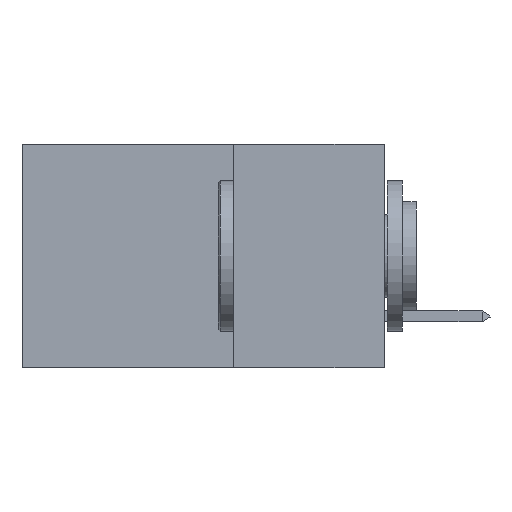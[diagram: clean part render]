
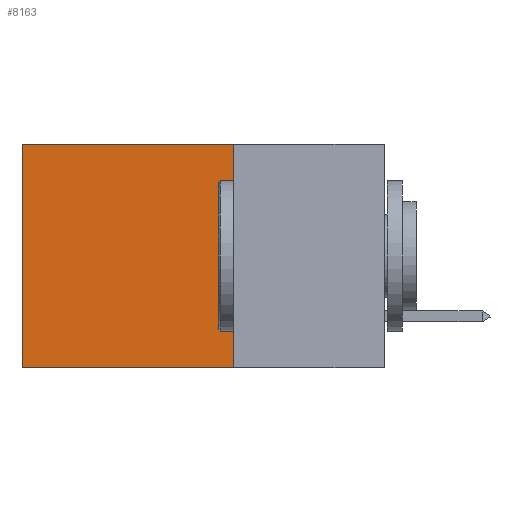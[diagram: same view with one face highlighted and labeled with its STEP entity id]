
A CAD part, left-side view. The second image highlights one B-rep face of the part: STEP entity #8163.
In plain terms, the highlighted planar face has unit normal (-1, 0, 0).
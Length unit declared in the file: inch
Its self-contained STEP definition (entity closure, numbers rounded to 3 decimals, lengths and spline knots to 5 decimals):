
#637 = CARTESIAN_POINT ( 'NONE',  ( 0.2875, 0.25, 0. ) ) ;
#3453 = PLANE ( 'NONE',  #29479 ) ;
#4338 = LINE ( 'NONE', #637, #24666 ) ;
#6359 = DIRECTION ( 'NONE',  ( 0., 0., -1. ) ) ;
#6366 = EDGE_CURVE ( 'NONE', #25277, #26230, #37629, .T. ) ;
#6501 = VECTOR ( 'NONE', #15849, 39.37008 ) ;
#6583 = CARTESIAN_POINT ( 'NONE',  ( 0.2875, 0.6, 0. ) ) ;
#7152 = ORIENTED_EDGE ( 'NONE', *, *, #24668, .T. ) ;
#7174 = CARTESIAN_POINT ( 'NONE',  ( 0.2875, 0.6, 0. ) ) ;
#8163 = ADVANCED_FACE ( 'NONE', ( #38604 ), #3453, .F. ) ;
#10788 = CARTESIAN_POINT ( 'NONE',  ( 0.2875, 0.6, -0.37 ) ) ;
#14595 = LINE ( 'NONE', #6583, #6501 ) ;
#15849 = DIRECTION ( 'NONE',  ( 0., 0., -1. ) ) ;
#18661 = VERTEX_POINT ( 'NONE', #21433 ) ;
#20724 = ORIENTED_EDGE ( 'NONE', *, *, #38554, .F. ) ;
#20881 = LINE ( 'NONE', #33372, #22767 ) ;
#21162 = DIRECTION ( 'NONE',  ( 0., 1., 0. ) ) ;
#21433 = CARTESIAN_POINT ( 'NONE',  ( 0.2875, 0.25, -0.37 ) ) ;
#22767 = VECTOR ( 'NONE', #21162, 39.37008 ) ;
#23547 = ORIENTED_EDGE ( 'NONE', *, *, #6366, .T. ) ;
#23652 = CARTESIAN_POINT ( 'NONE',  ( 0.2875, 0.25, 0. ) ) ;
#24072 = EDGE_LOOP ( 'NONE', ( #7152, #20724, #25419, #23547 ) ) ;
#24666 = VECTOR ( 'NONE', #30499, 39.37008 ) ;
#24668 = EDGE_CURVE ( 'NONE', #26230, #38959, #14595, .T. ) ;
#25277 = VERTEX_POINT ( 'NONE', #23652 ) ;
#25419 = ORIENTED_EDGE ( 'NONE', *, *, #38098, .F. ) ;
#26230 = VERTEX_POINT ( 'NONE', #7174 ) ;
#26471 = CARTESIAN_POINT ( 'NONE',  ( 0.2875, 0.25, 0. ) ) ;
#29226 = DIRECTION ( 'NONE',  ( 0., 1., 0. ) ) ;
#29479 = AXIS2_PLACEMENT_3D ( 'NONE', #30252, #39161, #6359 ) ;
#30252 = CARTESIAN_POINT ( 'NONE',  ( 0.2875, 0.25, 0. ) ) ;
#30499 = DIRECTION ( 'NONE',  ( 0., 0., -1. ) ) ;
#33372 = CARTESIAN_POINT ( 'NONE',  ( 0.2875, 0.25, -0.37 ) ) ;
#35287 = VECTOR ( 'NONE', #29226, 39.37008 ) ;
#37629 = LINE ( 'NONE', #26471, #35287 ) ;
#38098 = EDGE_CURVE ( 'NONE', #25277, #18661, #4338, .T. ) ;
#38554 = EDGE_CURVE ( 'NONE', #18661, #38959, #20881, .T. ) ;
#38604 = FACE_OUTER_BOUND ( 'NONE', #24072, .T. ) ;
#38959 = VERTEX_POINT ( 'NONE', #10788 ) ;
#39161 = DIRECTION ( 'NONE',  ( 1., 0., 0. ) ) ;
